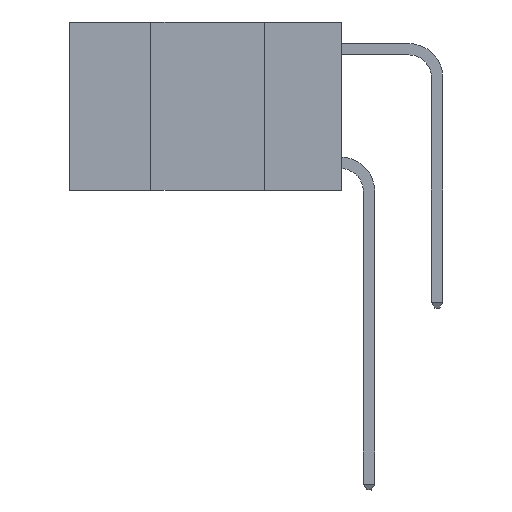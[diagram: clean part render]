
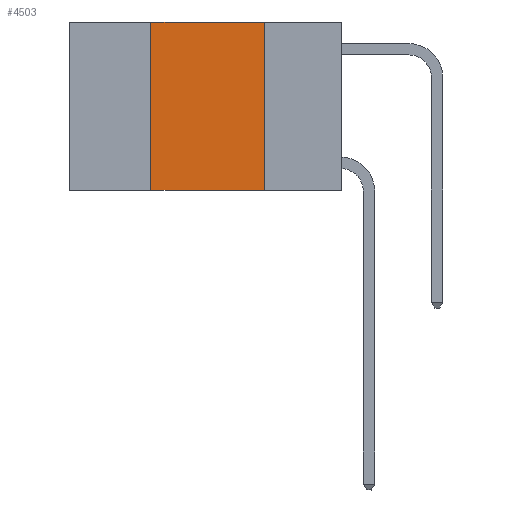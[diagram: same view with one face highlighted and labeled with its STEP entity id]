
A CAD part, left-side view. The second image highlights one B-rep face of the part: STEP entity #4503.
In plain terms, the highlighted planar face has unit normal (-1, 0, 0).
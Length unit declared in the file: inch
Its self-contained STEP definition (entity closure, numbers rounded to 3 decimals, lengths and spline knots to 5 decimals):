
#136 = CARTESIAN_POINT ( 'NONE',  ( 0., 0.17, -0.37 ) ) ;
#463 = DIRECTION ( 'NONE',  ( 0., -1., 0. ) ) ;
#940 = CARTESIAN_POINT ( 'NONE',  ( 0., 0.6, 0. ) ) ;
#1450 = LINE ( 'NONE', #12856, #17947 ) ;
#1531 = LINE ( 'NONE', #18868, #12921 ) ;
#1655 = ORIENTED_EDGE ( 'NONE', *, *, #6761, .F. ) ;
#2711 = ORIENTED_EDGE ( 'NONE', *, *, #11783, .F. ) ;
#2916 = AXIS2_PLACEMENT_3D ( 'NONE', #940, #12912, #4216 ) ;
#3197 = VECTOR ( 'NONE', #9343, 39.37008 ) ;
#4216 = DIRECTION ( 'NONE',  ( 0., 0., -1. ) ) ;
#4503 = ADVANCED_FACE ( 'NONE', ( #8889 ), #11474, .F. ) ;
#5627 = DIRECTION ( 'NONE',  ( 0., 0., -1. ) ) ;
#5766 = ORIENTED_EDGE ( 'NONE', *, *, #8722, .F. ) ;
#5790 = EDGE_CURVE ( 'NONE', #6454, #13137, #13391, .T. ) ;
#6151 = VECTOR ( 'NONE', #463, 39.37008 ) ;
#6454 = VERTEX_POINT ( 'NONE', #12666 ) ;
#6761 = EDGE_CURVE ( 'NONE', #6454, #10159, #1531, .T. ) ;
#7115 = LINE ( 'NONE', #16454, #3197 ) ;
#7276 = DIRECTION ( 'NONE',  ( 0., 0., 1. ) ) ;
#8128 = CARTESIAN_POINT ( 'NONE',  ( 0., 0.6, -0.37 ) ) ;
#8722 = EDGE_CURVE ( 'NONE', #11587, #13137, #1450, .T. ) ;
#8889 = FACE_OUTER_BOUND ( 'NONE', #9636, .T. ) ;
#9343 = DIRECTION ( 'NONE',  ( 0., -1., 0. ) ) ;
#9636 = EDGE_LOOP ( 'NONE', ( #5766, #2711, #1655, #17882 ) ) ;
#10159 = VERTEX_POINT ( 'NONE', #16079 ) ;
#11474 = PLANE ( 'NONE',  #2916 ) ;
#11587 = VERTEX_POINT ( 'NONE', #16106 ) ;
#11783 = EDGE_CURVE ( 'NONE', #10159, #11587, #7115, .T. ) ;
#12666 = CARTESIAN_POINT ( 'NONE',  ( 0., 0.42, -0.37 ) ) ;
#12856 = CARTESIAN_POINT ( 'NONE',  ( 0., 0.17, 0. ) ) ;
#12912 = DIRECTION ( 'NONE',  ( 1., 0., 0. ) ) ;
#12921 = VECTOR ( 'NONE', #7276, 39.37008 ) ;
#13137 = VERTEX_POINT ( 'NONE', #136 ) ;
#13391 = LINE ( 'NONE', #8128, #6151 ) ;
#16079 = CARTESIAN_POINT ( 'NONE',  ( 0., 0.42, 0. ) ) ;
#16106 = CARTESIAN_POINT ( 'NONE',  ( 0., 0.17, 0. ) ) ;
#16454 = CARTESIAN_POINT ( 'NONE',  ( 0., 0.6, 0. ) ) ;
#17882 = ORIENTED_EDGE ( 'NONE', *, *, #5790, .T. ) ;
#17947 = VECTOR ( 'NONE', #5627, 39.37008 ) ;
#18868 = CARTESIAN_POINT ( 'NONE',  ( 0., 0.42, 0. ) ) ;
